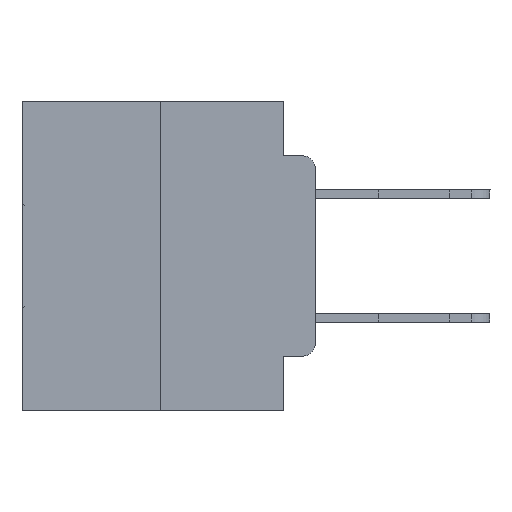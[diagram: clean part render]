
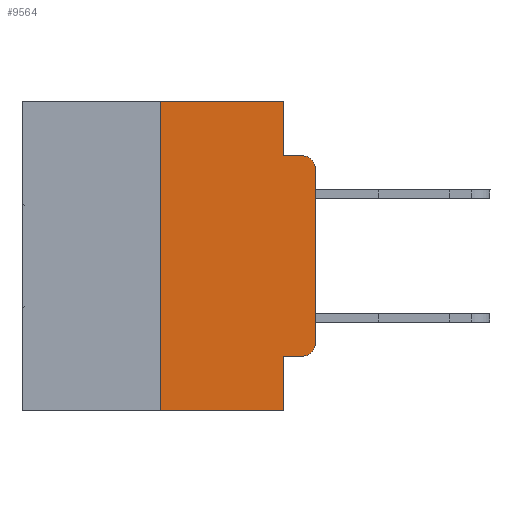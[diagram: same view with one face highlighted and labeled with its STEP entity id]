
A CAD part, left-side view. The second image highlights one B-rep face of the part: STEP entity #9564.
In plain terms, the highlighted planar face has unit normal (-1, 0, 0).
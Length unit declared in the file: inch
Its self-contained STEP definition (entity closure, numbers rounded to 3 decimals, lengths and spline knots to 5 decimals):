
#221 = ORIENTED_EDGE ( 'NONE', *, *, #29868, .T. ) ;
#634 = CARTESIAN_POINT ( 'NONE',  ( 0., 0.051, 0. ) ) ;
#744 = DIRECTION ( 'NONE',  ( 0., 0., -1. ) ) ;
#922 = EDGE_CURVE ( 'NONE', #15441, #22964, #17089, .T. ) ;
#1206 = DIRECTION ( 'NONE',  ( 0., 0., -1. ) ) ;
#1969 = VERTEX_POINT ( 'NONE', #19259 ) ;
#2022 = ORIENTED_EDGE ( 'NONE', *, *, #22452, .T. ) ;
#2198 = LINE ( 'NONE', #18899, #13375 ) ;
#2371 = LINE ( 'NONE', #7190, #11084 ) ;
#2512 = CARTESIAN_POINT ( 'NONE',  ( 0., 0.02, -0.1085 ) ) ;
#3109 = EDGE_CURVE ( 'NONE', #22964, #12936, #16358, .T. ) ;
#3351 = CARTESIAN_POINT ( 'NONE',  ( 0., 0.051, -0.4115 ) ) ;
#4190 = LINE ( 'NONE', #11670, #6316 ) ;
#4854 = CARTESIAN_POINT ( 'NONE',  ( 0., 0.051, -0.4115 ) ) ;
#5907 = CARTESIAN_POINT ( 'NONE',  ( 0., 0.02, -0.3915 ) ) ;
#6316 = VECTOR ( 'NONE', #21201, 39.37008 ) ;
#6886 = DIRECTION ( 'NONE',  ( 0., 0., -1. ) ) ;
#7012 = CARTESIAN_POINT ( 'NONE',  ( 0., 0.02, -0.4115 ) ) ;
#7178 = CARTESIAN_POINT ( 'NONE',  ( 0., 0.25, -0.5 ) ) ;
#7190 = CARTESIAN_POINT ( 'NONE',  ( 0., 0., 0. ) ) ;
#8025 = DIRECTION ( 'NONE',  ( 0., 0., 1. ) ) ;
#8220 = CIRCLE ( 'NONE', #8740, 0.02 ) ;
#8312 = CARTESIAN_POINT ( 'NONE',  ( 0., 0.25, 0. ) ) ;
#8351 = EDGE_CURVE ( 'NONE', #15441, #1969, #16115, .T. ) ;
#8740 = AXIS2_PLACEMENT_3D ( 'NONE', #2512, #21086, #6886 ) ;
#9174 = VERTEX_POINT ( 'NONE', #8312 ) ;
#9207 = FACE_OUTER_BOUND ( 'NONE', #30749, .T. ) ;
#9465 = CARTESIAN_POINT ( 'NONE',  ( 0., 0., -0.1085 ) ) ;
#9564 = ADVANCED_FACE ( 'NONE', ( #9207 ), #18724, .F. ) ;
#9772 = VECTOR ( 'NONE', #24600, 39.37008 ) ;
#10071 = VERTEX_POINT ( 'NONE', #14874 ) ;
#10211 = LINE ( 'NONE', #24439, #10910 ) ;
#10453 = LINE ( 'NONE', #634, #17138 ) ;
#10910 = VECTOR ( 'NONE', #8025, 39.37008 ) ;
#11084 = VECTOR ( 'NONE', #19060, 39.37008 ) ;
#11670 = CARTESIAN_POINT ( 'NONE',  ( 0., 0.473, 0. ) ) ;
#11776 = ORIENTED_EDGE ( 'NONE', *, *, #29147, .F. ) ;
#12216 = EDGE_CURVE ( 'NONE', #14065, #10071, #2198, .T. ) ;
#12376 = ORIENTED_EDGE ( 'NONE', *, *, #23965, .F. ) ;
#12936 = VERTEX_POINT ( 'NONE', #20852 ) ;
#13375 = VECTOR ( 'NONE', #28456, 39.37008 ) ;
#14056 = DIRECTION ( 'NONE',  ( 0., -1., 0. ) ) ;
#14065 = VERTEX_POINT ( 'NONE', #16836 ) ;
#14131 = EDGE_CURVE ( 'NONE', #15490, #1969, #30632, .T. ) ;
#14874 = CARTESIAN_POINT ( 'NONE',  ( 0., 0.02, -0.0885 ) ) ;
#15413 = DIRECTION ( 'NONE',  ( -1., 0., 0. ) ) ;
#15441 = VERTEX_POINT ( 'NONE', #4854 ) ;
#15490 = VERTEX_POINT ( 'NONE', #7178 ) ;
#15520 = VERTEX_POINT ( 'NONE', #19193 ) ;
#15795 = AXIS2_PLACEMENT_3D ( 'NONE', #16532, #29192, #744 ) ;
#16115 = LINE ( 'NONE', #16431, #30252 ) ;
#16358 = CIRCLE ( 'NONE', #22351, 0.02 ) ;
#16431 = CARTESIAN_POINT ( 'NONE',  ( 0., 0.051, 0. ) ) ;
#16532 = CARTESIAN_POINT ( 'NONE',  ( 0., 0.473, 0. ) ) ;
#16836 = CARTESIAN_POINT ( 'NONE',  ( 0., 0.051, -0.0885 ) ) ;
#17089 = LINE ( 'NONE', #3351, #9772 ) ;
#17138 = VECTOR ( 'NONE', #26565, 39.37008 ) ;
#18137 = ORIENTED_EDGE ( 'NONE', *, *, #12216, .F. ) ;
#18275 = ORIENTED_EDGE ( 'NONE', *, *, #922, .T. ) ;
#18652 = ORIENTED_EDGE ( 'NONE', *, *, #8351, .F. ) ;
#18724 = PLANE ( 'NONE',  #15795 ) ;
#18899 = CARTESIAN_POINT ( 'NONE',  ( 0., 0.051, -0.0885 ) ) ;
#19060 = DIRECTION ( 'NONE',  ( 0., 0., 1. ) ) ;
#19193 = CARTESIAN_POINT ( 'NONE',  ( 0., 0.051, 0. ) ) ;
#19231 = VERTEX_POINT ( 'NONE', #9465 ) ;
#19259 = CARTESIAN_POINT ( 'NONE',  ( 0., 0.051, -0.5 ) ) ;
#19525 = ORIENTED_EDGE ( 'NONE', *, *, #3109, .T. ) ;
#20773 = ORIENTED_EDGE ( 'NONE', *, *, #28467, .F. ) ;
#20852 = CARTESIAN_POINT ( 'NONE',  ( 0., 0., -0.3915 ) ) ;
#21070 = CARTESIAN_POINT ( 'NONE',  ( 0., 0.473, -0.5 ) ) ;
#21086 = DIRECTION ( 'NONE',  ( -1., 0., 0. ) ) ;
#21201 = DIRECTION ( 'NONE',  ( 0., -1., 0. ) ) ;
#22351 = AXIS2_PLACEMENT_3D ( 'NONE', #5907, #15413, #1206 ) ;
#22452 = EDGE_CURVE ( 'NONE', #12936, #19231, #2371, .T. ) ;
#22964 = VERTEX_POINT ( 'NONE', #7012 ) ;
#23617 = DIRECTION ( 'NONE',  ( 0., 0., -1. ) ) ;
#23950 = VECTOR ( 'NONE', #14056, 39.37008 ) ;
#23965 = EDGE_CURVE ( 'NONE', #15520, #14065, #10453, .T. ) ;
#24439 = CARTESIAN_POINT ( 'NONE',  ( 0., 0.25, 0. ) ) ;
#24600 = DIRECTION ( 'NONE',  ( 0., -1., 0. ) ) ;
#25303 = ORIENTED_EDGE ( 'NONE', *, *, #14131, .T. ) ;
#26565 = DIRECTION ( 'NONE',  ( 0., 0., -1. ) ) ;
#28456 = DIRECTION ( 'NONE',  ( 0., -1., 0. ) ) ;
#28467 = EDGE_CURVE ( 'NONE', #9174, #15520, #4190, .T. ) ;
#29147 = EDGE_CURVE ( 'NONE', #15490, #9174, #10211, .T. ) ;
#29192 = DIRECTION ( 'NONE',  ( 1., 0., 0. ) ) ;
#29868 = EDGE_CURVE ( 'NONE', #19231, #10071, #8220, .T. ) ;
#30252 = VECTOR ( 'NONE', #23617, 39.37008 ) ;
#30632 = LINE ( 'NONE', #21070, #23950 ) ;
#30749 = EDGE_LOOP ( 'NONE', ( #2022, #221, #18137, #12376, #20773, #11776, #25303, #18652, #18275, #19525 ) ) ;
